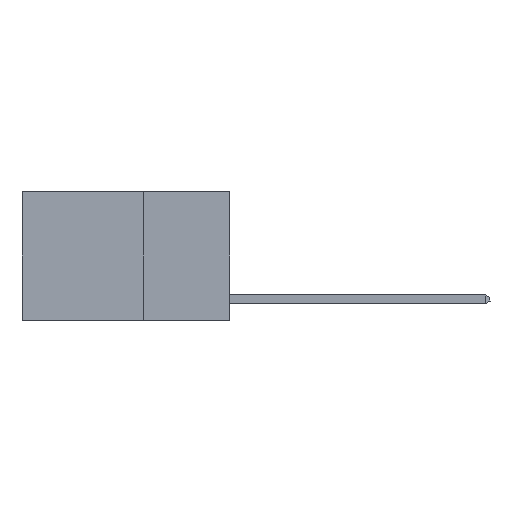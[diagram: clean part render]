
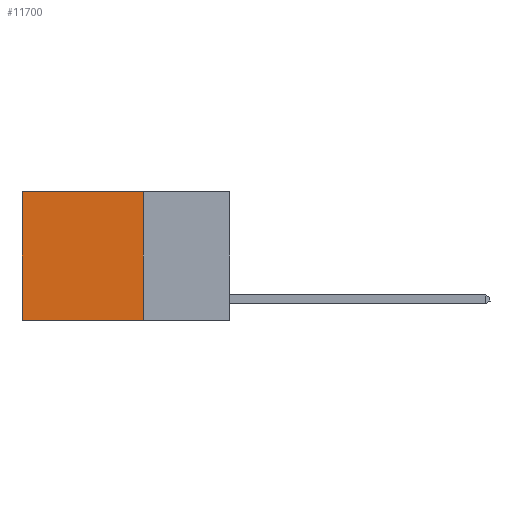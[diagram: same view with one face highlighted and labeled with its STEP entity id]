
A CAD part, left-side view. The second image highlights one B-rep face of the part: STEP entity #11700.
In plain terms, the highlighted planar face has unit normal (-1, 0, 0).
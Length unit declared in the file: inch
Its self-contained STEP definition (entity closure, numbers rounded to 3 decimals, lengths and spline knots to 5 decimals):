
#3 = FACE_OUTER_BOUND ( 'NONE', #5668, .T. ) ;
#298 = CARTESIAN_POINT ( 'NONE',  ( 0.2625, 0.6, 0. ) ) ;
#306 = DIRECTION ( 'NONE',  ( 0., 0., -1. ) ) ;
#486 = LINE ( 'NONE', #6685, #8949 ) ;
#529 = DIRECTION ( 'NONE',  ( 1., 0., 0. ) ) ;
#926 = AXIS2_PLACEMENT_3D ( 'NONE', #7002, #529, #8006 ) ;
#1259 = VERTEX_POINT ( 'NONE', #4220 ) ;
#1726 = ORIENTED_EDGE ( 'NONE', *, *, #12741, .F. ) ;
#2344 = DIRECTION ( 'NONE',  ( 0., 1., 0. ) ) ;
#3334 = EDGE_CURVE ( 'NONE', #1259, #12541, #486, .T. ) ;
#4220 = CARTESIAN_POINT ( 'NONE',  ( 0.2625, 0.25, -0.37 ) ) ;
#4428 = LINE ( 'NONE', #4661, #6587 ) ;
#4476 = ORIENTED_EDGE ( 'NONE', *, *, #11409, .T. ) ;
#4661 = CARTESIAN_POINT ( 'NONE',  ( 0.2625, 0.25, 0. ) ) ;
#4869 = PLANE ( 'NONE',  #926 ) ;
#4967 = VECTOR ( 'NONE', #8585, 39.37008 ) ;
#5058 = VERTEX_POINT ( 'NONE', #5898 ) ;
#5668 = EDGE_LOOP ( 'NONE', ( #12041, #9748, #1726, #4476 ) ) ;
#5775 = LINE ( 'NONE', #298, #8487 ) ;
#5898 = CARTESIAN_POINT ( 'NONE',  ( 0.2625, 0.25, 0. ) ) ;
#6537 = CARTESIAN_POINT ( 'NONE',  ( 0.2625, 0.25, 0. ) ) ;
#6587 = VECTOR ( 'NONE', #306, 39.37008 ) ;
#6685 = CARTESIAN_POINT ( 'NONE',  ( 0.2625, 0.25, -0.37 ) ) ;
#7002 = CARTESIAN_POINT ( 'NONE',  ( 0.2625, 0.25, 0. ) ) ;
#7069 = LINE ( 'NONE', #6537, #4967 ) ;
#7547 = VERTEX_POINT ( 'NONE', #8982 ) ;
#7795 = DIRECTION ( 'NONE',  ( 0., 0., -1. ) ) ;
#8006 = DIRECTION ( 'NONE',  ( 0., 0., -1. ) ) ;
#8487 = VECTOR ( 'NONE', #7795, 39.37008 ) ;
#8585 = DIRECTION ( 'NONE',  ( 0., 1., 0. ) ) ;
#8949 = VECTOR ( 'NONE', #2344, 39.37008 ) ;
#8982 = CARTESIAN_POINT ( 'NONE',  ( 0.2625, 0.6, 0. ) ) ;
#9748 = ORIENTED_EDGE ( 'NONE', *, *, #3334, .F. ) ;
#10095 = CARTESIAN_POINT ( 'NONE',  ( 0.2625, 0.6, -0.37 ) ) ;
#10929 = EDGE_CURVE ( 'NONE', #7547, #12541, #5775, .T. ) ;
#11409 = EDGE_CURVE ( 'NONE', #5058, #7547, #7069, .T. ) ;
#11700 = ADVANCED_FACE ( 'NONE', ( #3 ), #4869, .F. ) ;
#12041 = ORIENTED_EDGE ( 'NONE', *, *, #10929, .T. ) ;
#12541 = VERTEX_POINT ( 'NONE', #10095 ) ;
#12741 = EDGE_CURVE ( 'NONE', #5058, #1259, #4428, .T. ) ;
